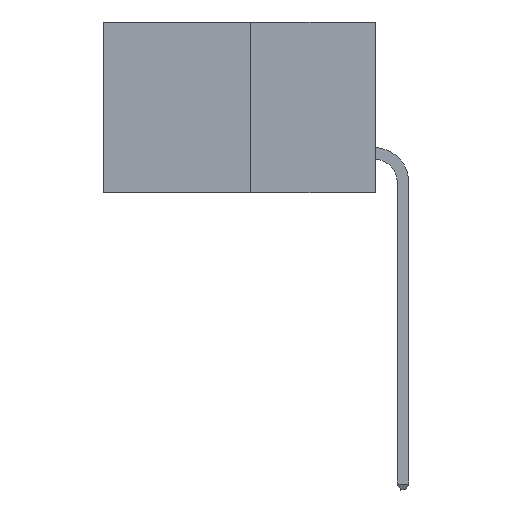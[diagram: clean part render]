
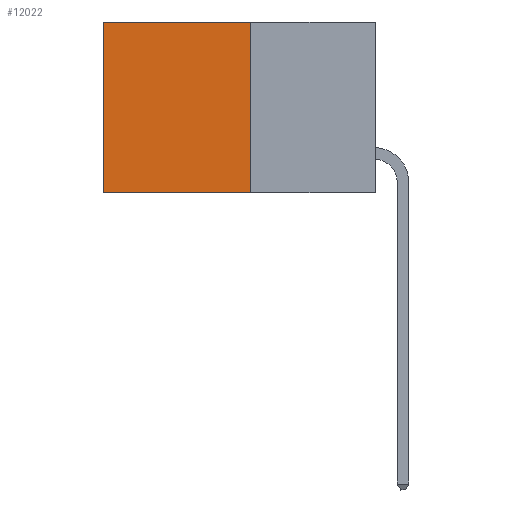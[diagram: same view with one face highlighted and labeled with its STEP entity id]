
A CAD part, left-side view. The second image highlights one B-rep face of the part: STEP entity #12022.
In plain terms, the highlighted planar face has unit normal (-1, 0, 0).
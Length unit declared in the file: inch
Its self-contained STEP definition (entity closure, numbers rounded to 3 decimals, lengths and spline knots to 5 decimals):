
#22 = VECTOR ( 'NONE', #21341, 39.37008 ) ;
#3855 = VERTEX_POINT ( 'NONE', #25582 ) ;
#5027 = EDGE_CURVE ( 'NONE', #20020, #3855, #24416, .T. ) ;
#7611 = CARTESIAN_POINT ( 'NONE',  ( 0.277, 0.59, -0.37 ) ) ;
#8961 = CARTESIAN_POINT ( 'NONE',  ( 0.277, 0.27, -0.37 ) ) ;
#9219 = EDGE_CURVE ( 'NONE', #20020, #15487, #26128, .T. ) ;
#10260 = AXIS2_PLACEMENT_3D ( 'NONE', #8961, #29344, #14125 ) ;
#12022 = ADVANCED_FACE ( 'NONE', ( #27613 ), #26887, .F. ) ;
#12330 = EDGE_CURVE ( 'NONE', #15487, #19291, #18069, .T. ) ;
#14125 = DIRECTION ( 'NONE',  ( 0., 0., -1. ) ) ;
#14696 = DIRECTION ( 'NONE',  ( 0., 1., 0. ) ) ;
#15487 = VERTEX_POINT ( 'NONE', #28063 ) ;
#15545 = CARTESIAN_POINT ( 'NONE',  ( 0.277, 0.27, 0. ) ) ;
#15612 = ORIENTED_EDGE ( 'NONE', *, *, #5027, .T. ) ;
#16999 = ORIENTED_EDGE ( 'NONE', *, *, #12330, .F. ) ;
#17265 = VECTOR ( 'NONE', #32917, 39.37008 ) ;
#17559 = VECTOR ( 'NONE', #14696, 39.37008 ) ;
#17952 = CARTESIAN_POINT ( 'NONE',  ( 0.277, 0.27, -0.37 ) ) ;
#18069 = LINE ( 'NONE', #17952, #17265 ) ;
#19004 = DIRECTION ( 'NONE',  ( 0., 0., -1. ) ) ;
#19291 = VERTEX_POINT ( 'NONE', #7611 ) ;
#20020 = VERTEX_POINT ( 'NONE', #15545 ) ;
#21341 = DIRECTION ( 'NONE',  ( 0., 0., -1. ) ) ;
#21468 = LINE ( 'NONE', #31267, #22 ) ;
#22374 = CARTESIAN_POINT ( 'NONE',  ( 0.277, 0.27, 0. ) ) ;
#22440 = EDGE_CURVE ( 'NONE', #3855, #19291, #21468, .T. ) ;
#22655 = EDGE_LOOP ( 'NONE', ( #29112, #16999, #32515, #15612 ) ) ;
#24416 = LINE ( 'NONE', #22374, #17559 ) ;
#25582 = CARTESIAN_POINT ( 'NONE',  ( 0.277, 0.59, 0. ) ) ;
#26128 = LINE ( 'NONE', #31511, #31863 ) ;
#26887 = PLANE ( 'NONE',  #10260 ) ;
#27613 = FACE_OUTER_BOUND ( 'NONE', #22655, .T. ) ;
#28063 = CARTESIAN_POINT ( 'NONE',  ( 0.277, 0.27, -0.37 ) ) ;
#29112 = ORIENTED_EDGE ( 'NONE', *, *, #22440, .T. ) ;
#29344 = DIRECTION ( 'NONE',  ( 1., 0., 0. ) ) ;
#31267 = CARTESIAN_POINT ( 'NONE',  ( 0.277, 0.59, -0.37 ) ) ;
#31511 = CARTESIAN_POINT ( 'NONE',  ( 0.277, 0.27, -0.37 ) ) ;
#31863 = VECTOR ( 'NONE', #19004, 39.37008 ) ;
#32515 = ORIENTED_EDGE ( 'NONE', *, *, #9219, .F. ) ;
#32917 = DIRECTION ( 'NONE',  ( 0., 1., 0. ) ) ;
